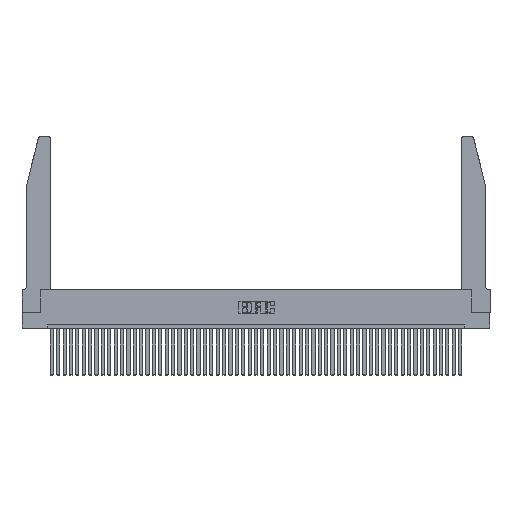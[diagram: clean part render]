
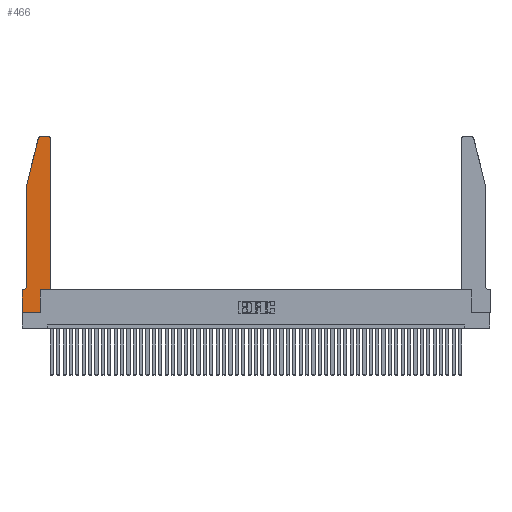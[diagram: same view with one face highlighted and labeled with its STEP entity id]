
A CAD part, top view. The second image highlights one B-rep face of the part: STEP entity #466.
In plain terms, the highlighted planar face has unit normal (0, 0, 1).
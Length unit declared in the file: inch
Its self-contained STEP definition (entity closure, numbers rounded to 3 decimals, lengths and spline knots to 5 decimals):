
#102 = VERTEX_POINT ( 'NONE', #15042 ) ;
#307 = DIRECTION ( 'NONE',  ( 0., 1., 0. ) ) ;
#466 = ADVANCED_FACE ( 'NONE', ( #46712 ), #17530, .T. ) ;
#505 = VERTEX_POINT ( 'NONE', #10123 ) ;
#2142 = ORIENTED_EDGE ( 'NONE', *, *, #17313, .T. ) ;
#2174 = ORIENTED_EDGE ( 'NONE', *, *, #43727, .T. ) ;
#2251 = DIRECTION ( 'NONE',  ( 1., 0., 0. ) ) ;
#2594 = LINE ( 'NONE', #48218, #22551 ) ;
#2687 = VECTOR ( 'NONE', #37393, 39.37008 ) ;
#4543 = VERTEX_POINT ( 'NONE', #29586 ) ;
#4669 = DIRECTION ( 'NONE',  ( -1., 0., 0. ) ) ;
#4951 = DIRECTION ( 'NONE',  ( -0.239, -0.971, 0. ) ) ;
#5261 = LINE ( 'NONE', #14987, #21585 ) ;
#6902 = VECTOR ( 'NONE', #49652, 39.37008 ) ;
#7283 = AXIS2_PLACEMENT_3D ( 'NONE', #34636, #19360, #15808 ) ;
#8275 = DIRECTION ( 'NONE',  ( 1., 0., 0. ) ) ;
#8439 = LINE ( 'NONE', #43834, #47410 ) ;
#9415 = EDGE_CURVE ( 'NONE', #28481, #38989, #31630, .T. ) ;
#9582 = EDGE_CURVE ( 'NONE', #44729, #4543, #24794, .T. ) ;
#10123 = CARTESIAN_POINT ( 'NONE',  ( 0.0755, 0.42, 0.37 ) ) ;
#10473 = CARTESIAN_POINT ( 'NONE',  ( 0.2865, 0., 0.37 ) ) ;
#11066 = DIRECTION ( 'NONE',  ( 0., 0., 1. ) ) ;
#11996 = EDGE_CURVE ( 'NONE', #38989, #16501, #33129, .T. ) ;
#12040 = VECTOR ( 'NONE', #307, 39.37008 ) ;
#14141 = AXIS2_PLACEMENT_3D ( 'NONE', #28989, #49277, #48793 ) ;
#14163 = EDGE_CURVE ( 'NONE', #4543, #28481, #43682, .T. ) ;
#14780 = ORIENTED_EDGE ( 'NONE', *, *, #11996, .T. ) ;
#14825 = VECTOR ( 'NONE', #4951, 39.37008 ) ;
#14987 = CARTESIAN_POINT ( 'NONE',  ( 0., 0., 0.37 ) ) ;
#15042 = CARTESIAN_POINT ( 'NONE',  ( 0.2865, 0.35, 0.37 ) ) ;
#15354 = CIRCLE ( 'NONE', #25415, 0.07 ) ;
#15808 = DIRECTION ( 'NONE',  ( 1., 0., 0. ) ) ;
#16501 = VERTEX_POINT ( 'NONE', #42494 ) ;
#16530 = EDGE_CURVE ( 'NONE', #18576, #47577, #32441, .T. ) ;
#16772 = CARTESIAN_POINT ( 'NONE',  ( 0.4505, 2.72, 0.37 ) ) ;
#16820 = DIRECTION ( 'NONE',  ( 1., 0., 0. ) ) ;
#17313 = EDGE_CURVE ( 'NONE', #34643, #102, #2594, .T. ) ;
#17446 = DIRECTION ( 'NONE',  ( -1., 0., 0. ) ) ;
#17530 = PLANE ( 'NONE',  #14141 ) ;
#17761 = ORIENTED_EDGE ( 'NONE', *, *, #25135, .T. ) ;
#18576 = VERTEX_POINT ( 'NONE', #21868 ) ;
#19360 = DIRECTION ( 'NONE',  ( 0., 0., 1. ) ) ;
#19532 = LINE ( 'NONE', #45748, #6902 ) ;
#20018 = EDGE_CURVE ( 'NONE', #16501, #505, #30844, .T. ) ;
#21585 = VECTOR ( 'NONE', #8275, 39.37008 ) ;
#21868 = CARTESIAN_POINT ( 'NONE',  ( 0.0055, 0.35, 0.37 ) ) ;
#21921 = ORIENTED_EDGE ( 'NONE', *, *, #14163, .T. ) ;
#22551 = VECTOR ( 'NONE', #24804, 39.37008 ) ;
#22858 = VECTOR ( 'NONE', #4669, 39.37008 ) ;
#23088 = VERTEX_POINT ( 'NONE', #31942 ) ;
#23196 = ORIENTED_EDGE ( 'NONE', *, *, #25451, .T. ) ;
#24615 = VERTEX_POINT ( 'NONE', #48249 ) ;
#24666 = VECTOR ( 'NONE', #39337, 39.37008 ) ;
#24794 = CIRCLE ( 'NONE', #7283, 0.03 ) ;
#24804 = DIRECTION ( 'NONE',  ( 0., 1., 0. ) ) ;
#25135 = EDGE_CURVE ( 'NONE', #102, #24615, #8439, .T. ) ;
#25415 = AXIS2_PLACEMENT_3D ( 'NONE', #33186, #49031, #17446 ) ;
#25451 = EDGE_CURVE ( 'NONE', #24615, #44729, #31544, .T. ) ;
#25903 = CARTESIAN_POINT ( 'NONE',  ( 0.0755, 0.35, 0.37 ) ) ;
#26403 = ORIENTED_EDGE ( 'NONE', *, *, #26697, .T. ) ;
#26697 = EDGE_CURVE ( 'NONE', #505, #18576, #15354, .T. ) ;
#27898 = CARTESIAN_POINT ( 'NONE',  ( 0.2605, 2.75, 0.37 ) ) ;
#28481 = VERTEX_POINT ( 'NONE', #33460 ) ;
#28989 = CARTESIAN_POINT ( 'NONE',  ( 0., 0.35, 0.37 ) ) ;
#29233 = EDGE_LOOP ( 'NONE', ( #21921, #32889, #14780, #37078, #26403, #50396, #2174, #47555, #2142, #17761, #23196, #37797 ) ) ;
#29586 = CARTESIAN_POINT ( 'NONE',  ( 0.4205, 2.75, 0.37 ) ) ;
#30844 = LINE ( 'NONE', #35390, #24666 ) ;
#31544 = LINE ( 'NONE', #34500, #12040 ) ;
#31630 = CIRCLE ( 'NONE', #38608, 0.03 ) ;
#31942 = CARTESIAN_POINT ( 'NONE',  ( 0., 0., 0.37 ) ) ;
#32441 = LINE ( 'NONE', #25903, #2687 ) ;
#32651 = EDGE_CURVE ( 'NONE', #23088, #34643, #5261, .T. ) ;
#32889 = ORIENTED_EDGE ( 'NONE', *, *, #9415, .T. ) ;
#33129 = LINE ( 'NONE', #39845, #14825 ) ;
#33186 = CARTESIAN_POINT ( 'NONE',  ( 0.0055, 0.42, 0.37 ) ) ;
#33460 = CARTESIAN_POINT ( 'NONE',  ( 0.284, 2.75, 0.37 ) ) ;
#34500 = CARTESIAN_POINT ( 'NONE',  ( 0.4505, 0.35, 0.37 ) ) ;
#34636 = CARTESIAN_POINT ( 'NONE',  ( 0.4205, 2.72, 0.37 ) ) ;
#34643 = VERTEX_POINT ( 'NONE', #10473 ) ;
#35390 = CARTESIAN_POINT ( 'NONE',  ( 0.0755, 2., 0.37 ) ) ;
#37078 = ORIENTED_EDGE ( 'NONE', *, *, #20018, .T. ) ;
#37393 = DIRECTION ( 'NONE',  ( -1., 0., 0. ) ) ;
#37797 = ORIENTED_EDGE ( 'NONE', *, *, #9582, .T. ) ;
#38608 = AXIS2_PLACEMENT_3D ( 'NONE', #46603, #11066, #2251 ) ;
#38989 = VERTEX_POINT ( 'NONE', #39357 ) ;
#39337 = DIRECTION ( 'NONE',  ( 0., -1., 0. ) ) ;
#39357 = CARTESIAN_POINT ( 'NONE',  ( 0.25487, 2.72718, 0.37 ) ) ;
#39845 = CARTESIAN_POINT ( 'NONE',  ( 0.0755, 2., 0.37 ) ) ;
#42197 = CARTESIAN_POINT ( 'NONE',  ( 0., 0.35, 0.37 ) ) ;
#42494 = CARTESIAN_POINT ( 'NONE',  ( 0.0755, 2., 0.37 ) ) ;
#43682 = LINE ( 'NONE', #27898, #22858 ) ;
#43727 = EDGE_CURVE ( 'NONE', #47577, #23088, #19532, .T. ) ;
#43834 = CARTESIAN_POINT ( 'NONE',  ( 0.4505, 0.35, 0.37 ) ) ;
#44729 = VERTEX_POINT ( 'NONE', #16772 ) ;
#45748 = CARTESIAN_POINT ( 'NONE',  ( 0., 0., 0.37 ) ) ;
#46603 = CARTESIAN_POINT ( 'NONE',  ( 0.284, 2.72, 0.37 ) ) ;
#46712 = FACE_OUTER_BOUND ( 'NONE', #29233, .T. ) ;
#47410 = VECTOR ( 'NONE', #16820, 39.37008 ) ;
#47555 = ORIENTED_EDGE ( 'NONE', *, *, #32651, .T. ) ;
#47577 = VERTEX_POINT ( 'NONE', #42197 ) ;
#48218 = CARTESIAN_POINT ( 'NONE',  ( 0.2865, 0.35, 0.37 ) ) ;
#48249 = CARTESIAN_POINT ( 'NONE',  ( 0.4505, 0.35, 0.37 ) ) ;
#48793 = DIRECTION ( 'NONE',  ( 1., 0., 0. ) ) ;
#49031 = DIRECTION ( 'NONE',  ( 0., 0., -1. ) ) ;
#49277 = DIRECTION ( 'NONE',  ( 0., 0., 1. ) ) ;
#49652 = DIRECTION ( 'NONE',  ( 0., -1., 0. ) ) ;
#50396 = ORIENTED_EDGE ( 'NONE', *, *, #16530, .T. ) ;
